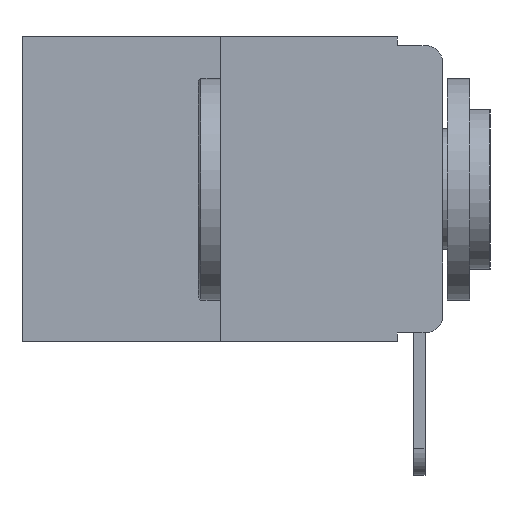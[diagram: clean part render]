
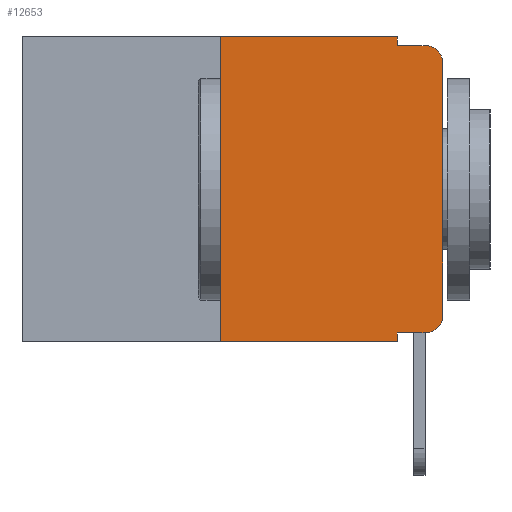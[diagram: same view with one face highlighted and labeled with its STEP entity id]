
A CAD part, left-side view. The second image highlights one B-rep face of the part: STEP entity #12653.
In plain terms, the highlighted planar face has unit normal (-1, 0, 0).
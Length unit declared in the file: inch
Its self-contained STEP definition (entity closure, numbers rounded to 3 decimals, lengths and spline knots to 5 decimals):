
#142 = ORIENTED_EDGE ( 'NONE', *, *, #1435, .F. ) ;
#161 = AXIS2_PLACEMENT_3D ( 'NONE', #7998, #5236, #11065 ) ;
#206 = VERTEX_POINT ( 'NONE', #2297 ) ;
#386 = CARTESIAN_POINT ( 'NONE',  ( 0., 0.473, 0. ) ) ;
#544 = VECTOR ( 'NONE', #16800, 39.37008 ) ;
#660 = EDGE_CURVE ( 'NONE', #17273, #1970, #8653, .T. ) ;
#1152 = VECTOR ( 'NONE', #9223, 39.37008 ) ;
#1156 = ORIENTED_EDGE ( 'NONE', *, *, #660, .T. ) ;
#1223 = DIRECTION ( 'NONE',  ( 0., -1., 0. ) ) ;
#1435 = EDGE_CURVE ( 'NONE', #12487, #4841, #16516, .T. ) ;
#1527 = VECTOR ( 'NONE', #14336, 39.37008 ) ;
#1602 = AXIS2_PLACEMENT_3D ( 'NONE', #386, #6118, #16403 ) ;
#1970 = VERTEX_POINT ( 'NONE', #6778 ) ;
#2156 = VERTEX_POINT ( 'NONE', #2159 ) ;
#2159 = CARTESIAN_POINT ( 'NONE',  ( 0., 0.02, -0.01 ) ) ;
#2297 = CARTESIAN_POINT ( 'NONE',  ( 0., 0.051, -0.333 ) ) ;
#3264 = CARTESIAN_POINT ( 'NONE',  ( 0., 0.051, -0.01 ) ) ;
#3406 = VERTEX_POINT ( 'NONE', #3264 ) ;
#3931 = LINE ( 'NONE', #4032, #13750 ) ;
#4032 = CARTESIAN_POINT ( 'NONE',  ( 0., 0.25, 0. ) ) ;
#4051 = DIRECTION ( 'NONE',  ( 0., 0., -1. ) ) ;
#4053 = DIRECTION ( 'NONE',  ( 0., 0., -1. ) ) ;
#4586 = CARTESIAN_POINT ( 'NONE',  ( 0., 0., -0.313 ) ) ;
#4841 = VERTEX_POINT ( 'NONE', #13817 ) ;
#5002 = EDGE_CURVE ( 'NONE', #7872, #12487, #3931, .T. ) ;
#5236 = DIRECTION ( 'NONE',  ( -1., 0., 0. ) ) ;
#5412 = ORIENTED_EDGE ( 'NONE', *, *, #17806, .F. ) ;
#5469 = DIRECTION ( 'NONE',  ( 0., 0., 1. ) ) ;
#5572 = VECTOR ( 'NONE', #8685, 39.37008 ) ;
#6013 = ORIENTED_EDGE ( 'NONE', *, *, #7178, .T. ) ;
#6118 = DIRECTION ( 'NONE',  ( 1., 0., 0. ) ) ;
#6778 = CARTESIAN_POINT ( 'NONE',  ( 0., 0., -0.03 ) ) ;
#6827 = CARTESIAN_POINT ( 'NONE',  ( 0., 0.02, -0.03 ) ) ;
#6962 = EDGE_CURVE ( 'NONE', #18082, #17273, #17937, .T. ) ;
#7084 = CARTESIAN_POINT ( 'NONE',  ( 0., 0.25, -0.343 ) ) ;
#7178 = EDGE_CURVE ( 'NONE', #206, #18082, #11159, .T. ) ;
#7227 = DIRECTION ( 'NONE',  ( 0., 0., 1. ) ) ;
#7244 = ORIENTED_EDGE ( 'NONE', *, *, #11892, .T. ) ;
#7816 = VECTOR ( 'NONE', #4051, 39.37008 ) ;
#7872 = VERTEX_POINT ( 'NONE', #7084 ) ;
#7998 = CARTESIAN_POINT ( 'NONE',  ( 0., 0.02, -0.313 ) ) ;
#8462 = CARTESIAN_POINT ( 'NONE',  ( 0., 0.051, -0.01 ) ) ;
#8653 = LINE ( 'NONE', #11526, #11223 ) ;
#8685 = DIRECTION ( 'NONE',  ( 0., -1., 0. ) ) ;
#8788 = EDGE_CURVE ( 'NONE', #3406, #2156, #15501, .T. ) ;
#9223 = DIRECTION ( 'NONE',  ( 0., 0., -1. ) ) ;
#9245 = ORIENTED_EDGE ( 'NONE', *, *, #13031, .T. ) ;
#10340 = FACE_OUTER_BOUND ( 'NONE', #11931, .T. ) ;
#10477 = AXIS2_PLACEMENT_3D ( 'NONE', #6827, #17221, #4053 ) ;
#10904 = CARTESIAN_POINT ( 'NONE',  ( 0., 0.473, 0. ) ) ;
#11065 = DIRECTION ( 'NONE',  ( 0., 0., -1. ) ) ;
#11159 = LINE ( 'NONE', #12794, #17659 ) ;
#11223 = VECTOR ( 'NONE', #7227, 39.37008 ) ;
#11526 = CARTESIAN_POINT ( 'NONE',  ( 0., 0., 0. ) ) ;
#11581 = CARTESIAN_POINT ( 'NONE',  ( 0., 0.25, 0. ) ) ;
#11892 = EDGE_CURVE ( 'NONE', #1970, #2156, #15400, .T. ) ;
#11931 = EDGE_LOOP ( 'NONE', ( #1156, #7244, #16074, #13832, #142, #16186, #9245, #5412, #6013, #12831 ) ) ;
#12487 = VERTEX_POINT ( 'NONE', #11581 ) ;
#12620 = CARTESIAN_POINT ( 'NONE',  ( 0., 0.051, -0.343 ) ) ;
#12653 = ADVANCED_FACE ( 'NONE', ( #10340 ), #15138, .F. ) ;
#12794 = CARTESIAN_POINT ( 'NONE',  ( 0., 0.051, -0.333 ) ) ;
#12831 = ORIENTED_EDGE ( 'NONE', *, *, #6962, .T. ) ;
#13031 = EDGE_CURVE ( 'NONE', #7872, #14152, #17466, .T. ) ;
#13641 = LINE ( 'NONE', #13733, #1152 ) ;
#13733 = CARTESIAN_POINT ( 'NONE',  ( 0., 0.051, 0. ) ) ;
#13750 = VECTOR ( 'NONE', #5469, 39.37008 ) ;
#13817 = CARTESIAN_POINT ( 'NONE',  ( 0., 0.051, 0. ) ) ;
#13832 = ORIENTED_EDGE ( 'NONE', *, *, #17939, .F. ) ;
#14152 = VERTEX_POINT ( 'NONE', #12620 ) ;
#14336 = DIRECTION ( 'NONE',  ( 0., -1., 0. ) ) ;
#15138 = PLANE ( 'NONE',  #1602 ) ;
#15400 = CIRCLE ( 'NONE', #10477, 0.02 ) ;
#15501 = LINE ( 'NONE', #8462, #1527 ) ;
#16016 = CARTESIAN_POINT ( 'NONE',  ( 0., 0.473, -0.343 ) ) ;
#16074 = ORIENTED_EDGE ( 'NONE', *, *, #8788, .F. ) ;
#16149 = CARTESIAN_POINT ( 'NONE',  ( 0., 0.02, -0.333 ) ) ;
#16186 = ORIENTED_EDGE ( 'NONE', *, *, #5002, .F. ) ;
#16403 = DIRECTION ( 'NONE',  ( 0., 0., -1. ) ) ;
#16516 = LINE ( 'NONE', #10904, #544 ) ;
#16800 = DIRECTION ( 'NONE',  ( 0., -1., 0. ) ) ;
#17218 = LINE ( 'NONE', #18841, #7816 ) ;
#17221 = DIRECTION ( 'NONE',  ( -1., 0., 0. ) ) ;
#17273 = VERTEX_POINT ( 'NONE', #4586 ) ;
#17466 = LINE ( 'NONE', #16016, #5572 ) ;
#17659 = VECTOR ( 'NONE', #1223, 39.37008 ) ;
#17806 = EDGE_CURVE ( 'NONE', #206, #14152, #13641, .T. ) ;
#17937 = CIRCLE ( 'NONE', #161, 0.02 ) ;
#17939 = EDGE_CURVE ( 'NONE', #4841, #3406, #17218, .T. ) ;
#18082 = VERTEX_POINT ( 'NONE', #16149 ) ;
#18841 = CARTESIAN_POINT ( 'NONE',  ( 0., 0.051, 0. ) ) ;
